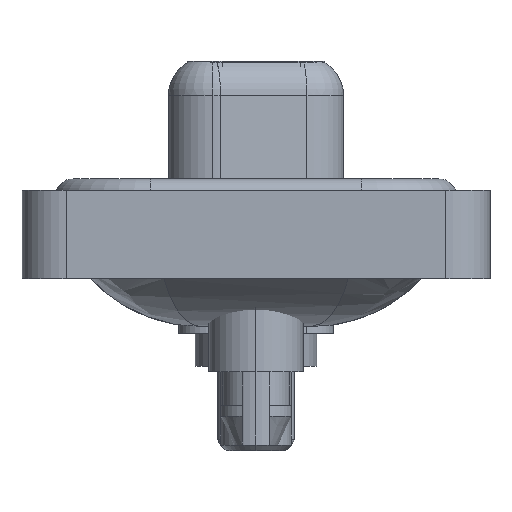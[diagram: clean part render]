
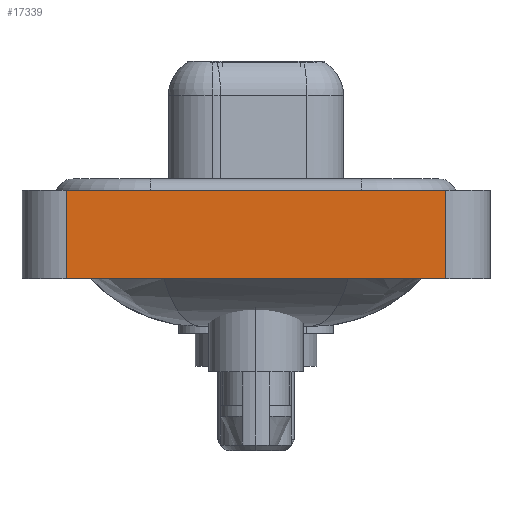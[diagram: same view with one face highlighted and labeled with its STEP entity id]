
A CAD part, left-side view. The second image highlights one B-rep face of the part: STEP entity #17339.
In plain terms, the highlighted planar face has unit normal (-1, 0, 0).
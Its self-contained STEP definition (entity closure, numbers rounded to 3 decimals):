
#68 = CARTESIAN_POINT ( 'NONE',  ( -7.35, -8.55, 0.4 ) ) ;
#895 = EDGE_LOOP ( 'NONE', ( #13269, #22980, #24292, #7260 ) ) ;
#963 = DIRECTION ( 'NONE',  ( 0., 0., 1. ) ) ;
#2362 = DIRECTION ( 'NONE',  ( -1., 0., 0. ) ) ;
#2827 = LINE ( 'NONE', #17011, #25876 ) ;
#2853 = VERTEX_POINT ( 'NONE', #17169 ) ;
#3078 = CARTESIAN_POINT ( 'NONE',  ( -7.35, -8.55, -3.6 ) ) ;
#3296 = EDGE_CURVE ( 'NONE', #2853, #25730, #21453, .T. ) ;
#3878 = CARTESIAN_POINT ( 'NONE',  ( -7.35, -8.55, 0.4 ) ) ;
#4082 = EDGE_CURVE ( 'NONE', #23581, #25730, #18099, .T. ) ;
#4805 = DIRECTION ( 'NONE',  ( 0., 0., 1. ) ) ;
#6052 = DIRECTION ( 'NONE',  ( 0., -1., 0. ) ) ;
#7260 = ORIENTED_EDGE ( 'NONE', *, *, #13192, .T. ) ;
#8104 = DIRECTION ( 'NONE',  ( 0., -1., 0. ) ) ;
#10253 = FACE_OUTER_BOUND ( 'NONE', #895, .T. ) ;
#10387 = DIRECTION ( 'NONE',  ( 0., 0., 1. ) ) ;
#11830 = LINE ( 'NONE', #23660, #15896 ) ;
#13192 = EDGE_CURVE ( 'NONE', #20579, #2853, #11830, .T. ) ;
#13269 = ORIENTED_EDGE ( 'NONE', *, *, #3296, .T. ) ;
#14317 = CARTESIAN_POINT ( 'NONE',  ( -7.35, -8.55, -3.6 ) ) ;
#15896 = VECTOR ( 'NONE', #6052, 1000. ) ;
#17011 = CARTESIAN_POINT ( 'NONE',  ( -7.35, 8.55, -3.6 ) ) ;
#17169 = CARTESIAN_POINT ( 'NONE',  ( -7.35, -8.55, -3.6 ) ) ;
#17339 = ADVANCED_FACE ( 'NONE', ( #10253 ), #18265, .T. ) ;
#17474 = AXIS2_PLACEMENT_3D ( 'NONE', #14317, #2362, #10387 ) ;
#17892 = EDGE_CURVE ( 'NONE', #20579, #23581, #2827, .T. ) ;
#18099 = LINE ( 'NONE', #68, #24039 ) ;
#18265 = PLANE ( 'NONE',  #17474 ) ;
#18308 = CARTESIAN_POINT ( 'NONE',  ( -7.35, 8.55, -3.6 ) ) ;
#20579 = VERTEX_POINT ( 'NONE', #18308 ) ;
#20621 = VECTOR ( 'NONE', #963, 1000. ) ;
#21453 = LINE ( 'NONE', #3078, #20621 ) ;
#21781 = CARTESIAN_POINT ( 'NONE',  ( -7.35, 8.55, 0.4 ) ) ;
#22980 = ORIENTED_EDGE ( 'NONE', *, *, #4082, .F. ) ;
#23581 = VERTEX_POINT ( 'NONE', #21781 ) ;
#23660 = CARTESIAN_POINT ( 'NONE',  ( -7.35, -8.55, -3.6 ) ) ;
#24039 = VECTOR ( 'NONE', #8104, 1000. ) ;
#24292 = ORIENTED_EDGE ( 'NONE', *, *, #17892, .F. ) ;
#25730 = VERTEX_POINT ( 'NONE', #3878 ) ;
#25876 = VECTOR ( 'NONE', #4805, 1000. ) ;
